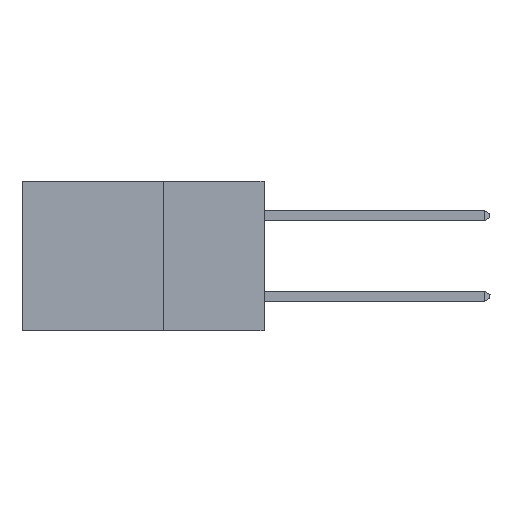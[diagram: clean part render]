
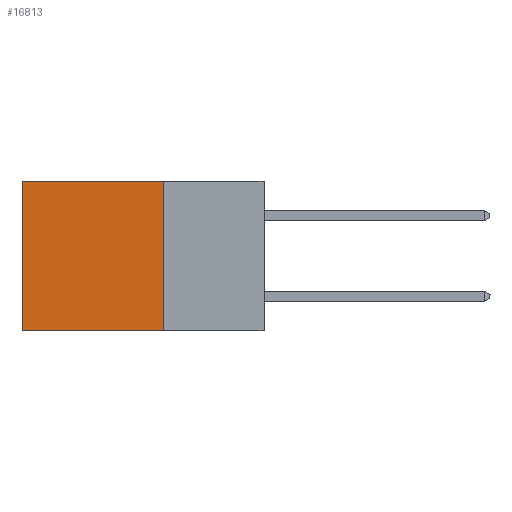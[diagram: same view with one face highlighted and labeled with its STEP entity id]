
A CAD part, left-side view. The second image highlights one B-rep face of the part: STEP entity #16813.
In plain terms, the highlighted planar face has unit normal (-1, 0, 0).
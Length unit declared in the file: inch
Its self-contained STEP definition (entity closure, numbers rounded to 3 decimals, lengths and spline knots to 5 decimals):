
#371 = VECTOR ( 'NONE', #2675, 39.37008 ) ;
#1290 = CARTESIAN_POINT ( 'NONE',  ( 0.298, 0.25, 0. ) ) ;
#2005 = VECTOR ( 'NONE', #17240, 39.37008 ) ;
#2675 = DIRECTION ( 'NONE',  ( 0., 1., 0. ) ) ;
#3235 = DIRECTION ( 'NONE',  ( 0., 0., -1. ) ) ;
#3754 = ORIENTED_EDGE ( 'NONE', *, *, #13542, .F. ) ;
#5513 = LINE ( 'NONE', #21312, #371 ) ;
#5781 = CARTESIAN_POINT ( 'NONE',  ( 0.298, 0.25, 0. ) ) ;
#6056 = CARTESIAN_POINT ( 'NONE',  ( 0.298, 0.6, 0. ) ) ;
#7098 = VERTEX_POINT ( 'NONE', #5781 ) ;
#7175 = LINE ( 'NONE', #6056, #2005 ) ;
#9386 = LINE ( 'NONE', #23103, #23468 ) ;
#10871 = DIRECTION ( 'NONE',  ( 0., 0., -1. ) ) ;
#12129 = VERTEX_POINT ( 'NONE', #19245 ) ;
#13542 = EDGE_CURVE ( 'NONE', #12129, #14964, #9386, .T. ) ;
#13614 = FACE_OUTER_BOUND ( 'NONE', #16425, .T. ) ;
#14315 = VERTEX_POINT ( 'NONE', #19697 ) ;
#14583 = DIRECTION ( 'NONE',  ( 1., 0., 0. ) ) ;
#14964 = VERTEX_POINT ( 'NONE', #23273 ) ;
#15560 = VECTOR ( 'NONE', #10871, 39.37008 ) ;
#15917 = DIRECTION ( 'NONE',  ( 0., 1., 0. ) ) ;
#16059 = EDGE_CURVE ( 'NONE', #14315, #14964, #7175, .T. ) ;
#16425 = EDGE_LOOP ( 'NONE', ( #18872, #3754, #23395, #22994 ) ) ;
#16813 = ADVANCED_FACE ( 'NONE', ( #13614 ), #18175, .F. ) ;
#17129 = AXIS2_PLACEMENT_3D ( 'NONE', #1290, #14583, #3235 ) ;
#17240 = DIRECTION ( 'NONE',  ( 0., 0., -1. ) ) ;
#18090 = EDGE_CURVE ( 'NONE', #7098, #12129, #19819, .T. ) ;
#18175 = PLANE ( 'NONE',  #17129 ) ;
#18872 = ORIENTED_EDGE ( 'NONE', *, *, #16059, .T. ) ;
#19245 = CARTESIAN_POINT ( 'NONE',  ( 0.298, 0.25, -0.37 ) ) ;
#19697 = CARTESIAN_POINT ( 'NONE',  ( 0.298, 0.6, 0. ) ) ;
#19819 = LINE ( 'NONE', #21876, #15560 ) ;
#21312 = CARTESIAN_POINT ( 'NONE',  ( 0.298, 0.25, 0. ) ) ;
#21676 = EDGE_CURVE ( 'NONE', #7098, #14315, #5513, .T. ) ;
#21876 = CARTESIAN_POINT ( 'NONE',  ( 0.298, 0.25, 0. ) ) ;
#22994 = ORIENTED_EDGE ( 'NONE', *, *, #21676, .T. ) ;
#23103 = CARTESIAN_POINT ( 'NONE',  ( 0.298, 0.25, -0.37 ) ) ;
#23273 = CARTESIAN_POINT ( 'NONE',  ( 0.298, 0.6, -0.37 ) ) ;
#23395 = ORIENTED_EDGE ( 'NONE', *, *, #18090, .F. ) ;
#23468 = VECTOR ( 'NONE', #15917, 39.37008 ) ;
